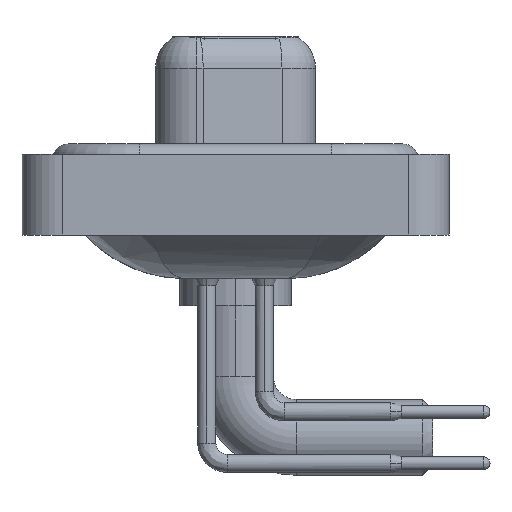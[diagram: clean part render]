
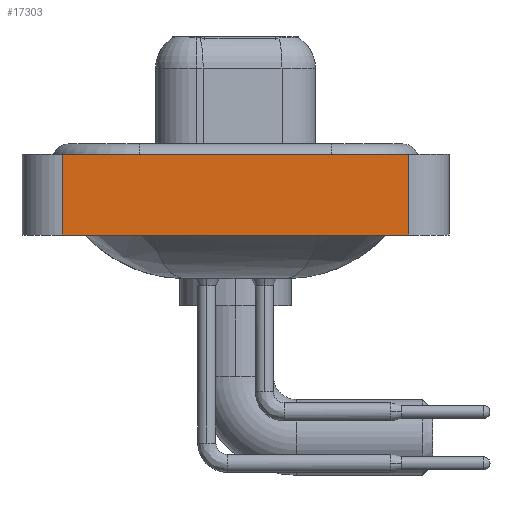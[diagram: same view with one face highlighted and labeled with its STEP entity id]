
A CAD part, left-side view. The second image highlights one B-rep face of the part: STEP entity #17303.
In plain terms, the highlighted planar face has unit normal (-1, 0, 0).
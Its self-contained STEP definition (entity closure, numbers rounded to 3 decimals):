
#369 = LINE ( 'NONE', #6576, #13857 ) ;
#448 = CARTESIAN_POINT ( 'NONE',  ( -7.25, -8.55, -3.6 ) ) ;
#738 = EDGE_CURVE ( 'NONE', #10040, #13628, #8971, .T. ) ;
#1252 = VECTOR ( 'NONE', #12082, 1000. ) ;
#1369 = LINE ( 'NONE', #7503, #9692 ) ;
#3127 = ORIENTED_EDGE ( 'NONE', *, *, #18296, .T. ) ;
#4682 = AXIS2_PLACEMENT_3D ( 'NONE', #14744, #17789, #12762 ) ;
#4724 = EDGE_CURVE ( 'NONE', #10040, #13319, #7916, .T. ) ;
#4978 = DIRECTION ( 'NONE',  ( 0., 0., 1. ) ) ;
#6416 = CARTESIAN_POINT ( 'NONE',  ( -7.25, -8.55, -3.6 ) ) ;
#6576 = CARTESIAN_POINT ( 'NONE',  ( -7.25, -8.55, -3.6 ) ) ;
#7503 = CARTESIAN_POINT ( 'NONE',  ( -7.25, -8.55, 0.4 ) ) ;
#7916 = LINE ( 'NONE', #6416, #14797 ) ;
#8251 = FACE_OUTER_BOUND ( 'NONE', #17119, .T. ) ;
#8971 = LINE ( 'NONE', #10572, #1252 ) ;
#9507 = CARTESIAN_POINT ( 'NONE',  ( -7.25, -8.55, 0.4 ) ) ;
#9692 = VECTOR ( 'NONE', #15494, 1000. ) ;
#10040 = VERTEX_POINT ( 'NONE', #15729 ) ;
#10572 = CARTESIAN_POINT ( 'NONE',  ( -7.25, 8.55, -3.6 ) ) ;
#12082 = DIRECTION ( 'NONE',  ( 0., 0., 1. ) ) ;
#12430 = VERTEX_POINT ( 'NONE', #9507 ) ;
#12489 = ORIENTED_EDGE ( 'NONE', *, *, #738, .F. ) ;
#12525 = DIRECTION ( 'NONE',  ( 0., -1., 0. ) ) ;
#12762 = DIRECTION ( 'NONE',  ( 0., 0., 1. ) ) ;
#13319 = VERTEX_POINT ( 'NONE', #448 ) ;
#13628 = VERTEX_POINT ( 'NONE', #16884 ) ;
#13857 = VECTOR ( 'NONE', #4978, 1000. ) ;
#14744 = CARTESIAN_POINT ( 'NONE',  ( -7.25, -8.55, -3.6 ) ) ;
#14797 = VECTOR ( 'NONE', #12525, 1000. ) ;
#15494 = DIRECTION ( 'NONE',  ( 0., -1., 0. ) ) ;
#15729 = CARTESIAN_POINT ( 'NONE',  ( -7.25, 8.55, -3.6 ) ) ;
#16155 = PLANE ( 'NONE',  #4682 ) ;
#16654 = ORIENTED_EDGE ( 'NONE', *, *, #18254, .F. ) ;
#16884 = CARTESIAN_POINT ( 'NONE',  ( -7.25, 8.55, 0.4 ) ) ;
#17119 = EDGE_LOOP ( 'NONE', ( #3127, #16654, #12489, #17450 ) ) ;
#17303 = ADVANCED_FACE ( 'NONE', ( #8251 ), #16155, .T. ) ;
#17450 = ORIENTED_EDGE ( 'NONE', *, *, #4724, .T. ) ;
#17789 = DIRECTION ( 'NONE',  ( -1., 0., 0. ) ) ;
#18254 = EDGE_CURVE ( 'NONE', #13628, #12430, #1369, .T. ) ;
#18296 = EDGE_CURVE ( 'NONE', #13319, #12430, #369, .T. ) ;
